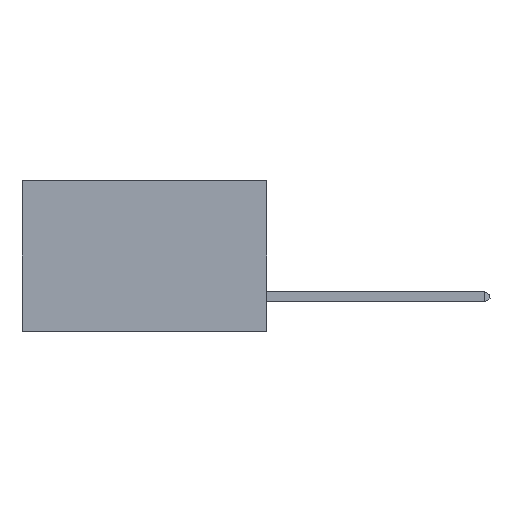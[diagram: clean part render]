
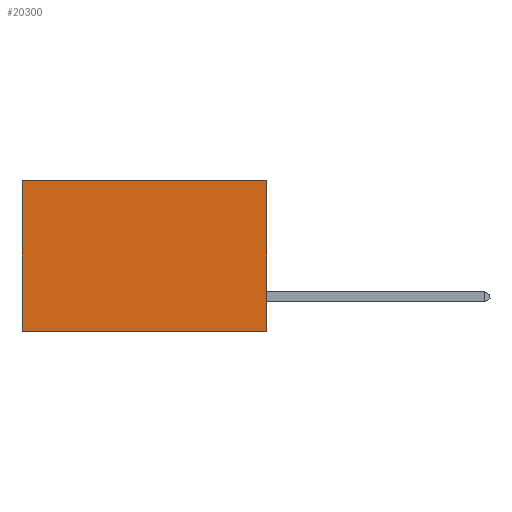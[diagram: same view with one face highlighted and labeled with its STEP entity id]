
A CAD part, left-side view. The second image highlights one B-rep face of the part: STEP entity #20300.
In plain terms, the highlighted planar face has unit normal (-1, 0, 0).
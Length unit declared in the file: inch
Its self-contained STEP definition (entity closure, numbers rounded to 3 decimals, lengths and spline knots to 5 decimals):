
#474 = CARTESIAN_POINT ( 'NONE',  ( 0.2875, 0.6, 0. ) ) ;
#2843 = VERTEX_POINT ( 'NONE', #21587 ) ;
#2925 = ORIENTED_EDGE ( 'NONE', *, *, #9691, .T. ) ;
#4384 = DIRECTION ( 'NONE',  ( 0., 1., 0. ) ) ;
#4605 = EDGE_CURVE ( 'NONE', #2843, #20489, #10320, .T. ) ;
#4854 = EDGE_CURVE ( 'NONE', #21151, #20489, #31635, .T. ) ;
#6104 = VECTOR ( 'NONE', #29377, 39.37008 ) ;
#6282 = CARTESIAN_POINT ( 'NONE',  ( 0.2875, 0., 0. ) ) ;
#7746 = EDGE_LOOP ( 'NONE', ( #33465, #29314, #20226, #2925 ) ) ;
#9087 = PLANE ( 'NONE',  #19423 ) ;
#9094 = DIRECTION ( 'NONE',  ( 0., 0., -1. ) ) ;
#9691 = EDGE_CURVE ( 'NONE', #32789, #2843, #13481, .T. ) ;
#10320 = LINE ( 'NONE', #474, #31241 ) ;
#11021 = CARTESIAN_POINT ( 'NONE',  ( 0.2875, 0., 0. ) ) ;
#11861 = CARTESIAN_POINT ( 'NONE',  ( 0.2875, 0., 0. ) ) ;
#13481 = LINE ( 'NONE', #21283, #6104 ) ;
#15845 = CARTESIAN_POINT ( 'NONE',  ( 0.2875, 0., -0.37 ) ) ;
#17095 = DIRECTION ( 'NONE',  ( 0., 0., -1. ) ) ;
#17339 = DIRECTION ( 'NONE',  ( 0., 0., -1. ) ) ;
#18165 = CARTESIAN_POINT ( 'NONE',  ( 0.2875, 0., -0.37 ) ) ;
#19423 = AXIS2_PLACEMENT_3D ( 'NONE', #11861, #33684, #17339 ) ;
#20226 = ORIENTED_EDGE ( 'NONE', *, *, #33646, .F. ) ;
#20300 = ADVANCED_FACE ( 'NONE', ( #22905 ), #9087, .F. ) ;
#20489 = VERTEX_POINT ( 'NONE', #26277 ) ;
#21151 = VERTEX_POINT ( 'NONE', #15845 ) ;
#21283 = CARTESIAN_POINT ( 'NONE',  ( 0.2875, 0., 0. ) ) ;
#21587 = CARTESIAN_POINT ( 'NONE',  ( 0.2875, 0.6, 0. ) ) ;
#21761 = LINE ( 'NONE', #6282, #35386 ) ;
#22905 = FACE_OUTER_BOUND ( 'NONE', #7746, .T. ) ;
#23570 = VECTOR ( 'NONE', #4384, 39.37008 ) ;
#26277 = CARTESIAN_POINT ( 'NONE',  ( 0.2875, 0.6, -0.37 ) ) ;
#29314 = ORIENTED_EDGE ( 'NONE', *, *, #4854, .F. ) ;
#29377 = DIRECTION ( 'NONE',  ( 0., 1., 0. ) ) ;
#31241 = VECTOR ( 'NONE', #17095, 39.37008 ) ;
#31635 = LINE ( 'NONE', #18165, #23570 ) ;
#32789 = VERTEX_POINT ( 'NONE', #11021 ) ;
#33465 = ORIENTED_EDGE ( 'NONE', *, *, #4605, .T. ) ;
#33646 = EDGE_CURVE ( 'NONE', #32789, #21151, #21761, .T. ) ;
#33684 = DIRECTION ( 'NONE',  ( 1., 0., 0. ) ) ;
#35386 = VECTOR ( 'NONE', #9094, 39.37008 ) ;
